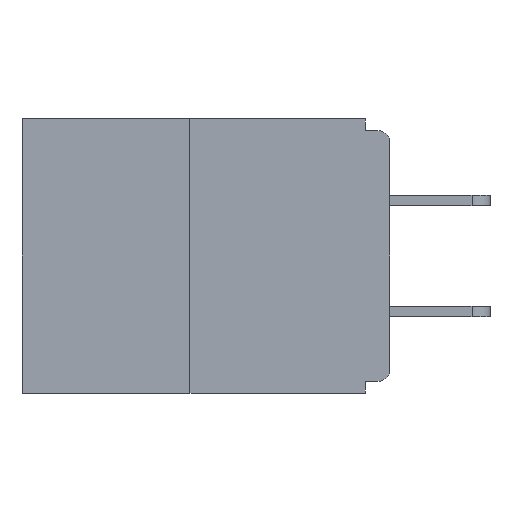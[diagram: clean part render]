
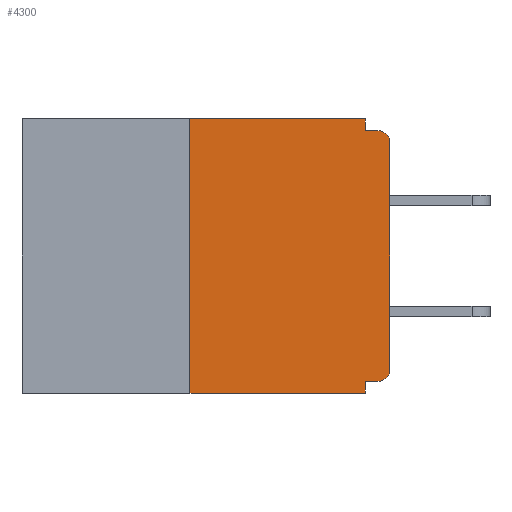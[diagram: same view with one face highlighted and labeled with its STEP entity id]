
A CAD part, left-side view. The second image highlights one B-rep face of the part: STEP entity #4300.
In plain terms, the highlighted planar face has unit normal (-1, 0, 0).
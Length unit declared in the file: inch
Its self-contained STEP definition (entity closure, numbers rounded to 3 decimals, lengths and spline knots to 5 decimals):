
#212 = ORIENTED_EDGE ( 'NONE', *, *, #11004, .F. ) ;
#461 = LINE ( 'NONE', #864, #18508 ) ;
#864 = CARTESIAN_POINT ( 'NONE',  ( 0., 0.031, -0.343 ) ) ;
#1145 = DIRECTION ( 'NONE',  ( 0., -1., 0. ) ) ;
#1168 = CARTESIAN_POINT ( 'NONE',  ( 0., 0.015, -0.015 ) ) ;
#1702 = CARTESIAN_POINT ( 'NONE',  ( 0., 0., 0. ) ) ;
#1809 = DIRECTION ( 'NONE',  ( -1., 0., 0. ) ) ;
#1932 = EDGE_CURVE ( 'NONE', #19353, #25639, #27072, .T. ) ;
#2348 = EDGE_CURVE ( 'NONE', #20827, #23894, #27017, .T. ) ;
#2424 = DIRECTION ( 'NONE',  ( 0., -1., 0. ) ) ;
#2434 = CARTESIAN_POINT ( 'NONE',  ( 0., 0.25, -0.343 ) ) ;
#2950 = CARTESIAN_POINT ( 'NONE',  ( 0., 0.25, 0. ) ) ;
#3819 = ORIENTED_EDGE ( 'NONE', *, *, #2348, .F. ) ;
#3878 = AXIS2_PLACEMENT_3D ( 'NONE', #12480, #25092, #20922 ) ;
#3898 = CARTESIAN_POINT ( 'NONE',  ( 0., 0.46, 0. ) ) ;
#3941 = PLANE ( 'NONE',  #4769 ) ;
#4210 = DIRECTION ( 'NONE',  ( 0., 0., -1. ) ) ;
#4300 = ADVANCED_FACE ( 'NONE', ( #25769 ), #3941, .F. ) ;
#4759 = VECTOR ( 'NONE', #1145, 39.37008 ) ;
#4760 = VECTOR ( 'NONE', #2424, 39.37008 ) ;
#4769 = AXIS2_PLACEMENT_3D ( 'NONE', #16512, #16594, #4210 ) ;
#4927 = CARTESIAN_POINT ( 'NONE',  ( 0., 0., -0.313 ) ) ;
#5844 = DIRECTION ( 'NONE',  ( 0., 0., -1. ) ) ;
#5907 = DIRECTION ( 'NONE',  ( 0., 0., 1. ) ) ;
#6014 = VECTOR ( 'NONE', #14987, 39.37008 ) ;
#7375 = EDGE_CURVE ( 'NONE', #9128, #18795, #22691, .T. ) ;
#7801 = VERTEX_POINT ( 'NONE', #22823 ) ;
#8497 = DIRECTION ( 'NONE',  ( 0., 0., 1. ) ) ;
#8779 = CIRCLE ( 'NONE', #12789, 0.015 ) ;
#9128 = VERTEX_POINT ( 'NONE', #2434 ) ;
#9601 = EDGE_LOOP ( 'NONE', ( #212, #13231, #23983, #22953, #25586, #14517, #23741, #26454, #3819, #25828 ) ) ;
#9951 = EDGE_CURVE ( 'NONE', #25639, #23894, #8779, .T. ) ;
#10365 = LINE ( 'NONE', #3898, #4760 ) ;
#10529 = CARTESIAN_POINT ( 'NONE',  ( 0., 0.031, 0. ) ) ;
#10691 = LINE ( 'NONE', #12521, #14294 ) ;
#10870 = CIRCLE ( 'NONE', #3878, 0.015 ) ;
#11002 = CARTESIAN_POINT ( 'NONE',  ( 0., 0., -0.03 ) ) ;
#11004 = EDGE_CURVE ( 'NONE', #18795, #15413, #10365, .T. ) ;
#11576 = CARTESIAN_POINT ( 'NONE',  ( 0., 0., -0.015 ) ) ;
#11607 = EDGE_CURVE ( 'NONE', #21538, #7801, #461, .T. ) ;
#12174 = CARTESIAN_POINT ( 'NONE',  ( 0., 0.015, -0.03 ) ) ;
#12361 = EDGE_CURVE ( 'NONE', #15413, #20827, #20793, .T. ) ;
#12480 = CARTESIAN_POINT ( 'NONE',  ( 0., 0.015, -0.313 ) ) ;
#12521 = CARTESIAN_POINT ( 'NONE',  ( 0., 0.46, -0.343 ) ) ;
#12789 = AXIS2_PLACEMENT_3D ( 'NONE', #12174, #1809, #5844 ) ;
#13231 = ORIENTED_EDGE ( 'NONE', *, *, #7375, .F. ) ;
#13451 = VECTOR ( 'NONE', #26062, 39.37008 ) ;
#13923 = EDGE_CURVE ( 'NONE', #23889, #21538, #16434, .T. ) ;
#14294 = VECTOR ( 'NONE', #20879, 39.37008 ) ;
#14517 = ORIENTED_EDGE ( 'NONE', *, *, #25969, .T. ) ;
#14634 = CARTESIAN_POINT ( 'NONE',  ( 0., 0.25, 0. ) ) ;
#14987 = DIRECTION ( 'NONE',  ( 0., 0., -1. ) ) ;
#15307 = VECTOR ( 'NONE', #5907, 39.37008 ) ;
#15413 = VERTEX_POINT ( 'NONE', #26890 ) ;
#15447 = DIRECTION ( 'NONE',  ( 0., 0., -1. ) ) ;
#15921 = CARTESIAN_POINT ( 'NONE',  ( 0., 0.015, -0.328 ) ) ;
#16434 = LINE ( 'NONE', #23957, #13451 ) ;
#16512 = CARTESIAN_POINT ( 'NONE',  ( 0., 0.46, 0. ) ) ;
#16594 = DIRECTION ( 'NONE',  ( 1., 0., 0. ) ) ;
#18508 = VECTOR ( 'NONE', #15447, 39.37008 ) ;
#18795 = VERTEX_POINT ( 'NONE', #2950 ) ;
#19353 = VERTEX_POINT ( 'NONE', #4927 ) ;
#19370 = CARTESIAN_POINT ( 'NONE',  ( 0., 0.031, -0.328 ) ) ;
#20793 = LINE ( 'NONE', #10529, #6014 ) ;
#20827 = VERTEX_POINT ( 'NONE', #25917 ) ;
#20879 = DIRECTION ( 'NONE',  ( 0., -1., 0. ) ) ;
#20922 = DIRECTION ( 'NONE',  ( 0., 0., -1. ) ) ;
#21240 = EDGE_CURVE ( 'NONE', #9128, #7801, #10691, .T. ) ;
#21538 = VERTEX_POINT ( 'NONE', #19370 ) ;
#22691 = LINE ( 'NONE', #14634, #25601 ) ;
#22823 = CARTESIAN_POINT ( 'NONE',  ( 0., 0.031, -0.343 ) ) ;
#22953 = ORIENTED_EDGE ( 'NONE', *, *, #11607, .F. ) ;
#23741 = ORIENTED_EDGE ( 'NONE', *, *, #1932, .T. ) ;
#23889 = VERTEX_POINT ( 'NONE', #15921 ) ;
#23894 = VERTEX_POINT ( 'NONE', #1168 ) ;
#23957 = CARTESIAN_POINT ( 'NONE',  ( 0., 0., -0.328 ) ) ;
#23983 = ORIENTED_EDGE ( 'NONE', *, *, #21240, .T. ) ;
#25092 = DIRECTION ( 'NONE',  ( -1., 0., 0. ) ) ;
#25586 = ORIENTED_EDGE ( 'NONE', *, *, #13923, .F. ) ;
#25601 = VECTOR ( 'NONE', #8497, 39.37008 ) ;
#25639 = VERTEX_POINT ( 'NONE', #11002 ) ;
#25769 = FACE_OUTER_BOUND ( 'NONE', #9601, .T. ) ;
#25828 = ORIENTED_EDGE ( 'NONE', *, *, #12361, .F. ) ;
#25917 = CARTESIAN_POINT ( 'NONE',  ( 0., 0.031, -0.015 ) ) ;
#25969 = EDGE_CURVE ( 'NONE', #23889, #19353, #10870, .T. ) ;
#26062 = DIRECTION ( 'NONE',  ( 0., 1., 0. ) ) ;
#26454 = ORIENTED_EDGE ( 'NONE', *, *, #9951, .T. ) ;
#26890 = CARTESIAN_POINT ( 'NONE',  ( 0., 0.031, 0. ) ) ;
#27017 = LINE ( 'NONE', #11576, #4759 ) ;
#27072 = LINE ( 'NONE', #1702, #15307 ) ;
